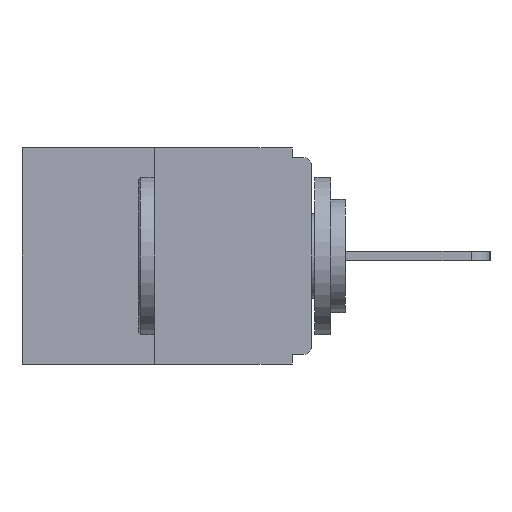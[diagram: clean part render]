
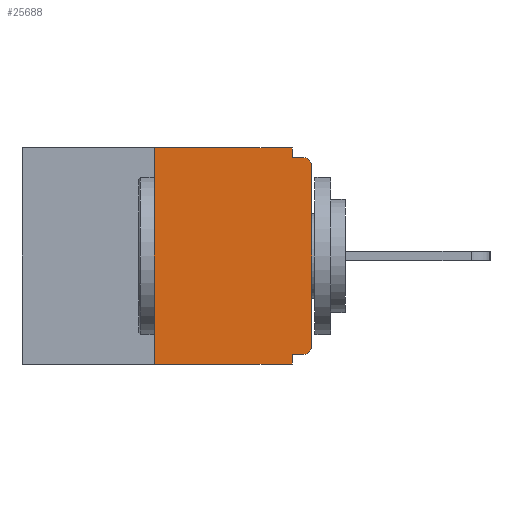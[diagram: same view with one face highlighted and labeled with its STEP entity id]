
A CAD part, left-side view. The second image highlights one B-rep face of the part: STEP entity #25688.
In plain terms, the highlighted planar face has unit normal (-1, 0, 0).
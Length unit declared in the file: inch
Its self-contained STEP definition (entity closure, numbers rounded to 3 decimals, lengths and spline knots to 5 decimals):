
#72 = DIRECTION ( 'NONE',  ( 0., 0., -1. ) ) ;
#695 = CARTESIAN_POINT ( 'NONE',  ( 0., 0.25, -0.343 ) ) ;
#706 = ORIENTED_EDGE ( 'NONE', *, *, #8228, .T. ) ;
#1074 = ORIENTED_EDGE ( 'NONE', *, *, #24626, .F. ) ;
#1727 = LINE ( 'NONE', #18703, #23089 ) ;
#2101 = DIRECTION ( 'NONE',  ( -1., 0., 0. ) ) ;
#2725 = DIRECTION ( 'NONE',  ( 0., -1., 0. ) ) ;
#3169 = DIRECTION ( 'NONE',  ( 0., -1., 0. ) ) ;
#3183 = AXIS2_PLACEMENT_3D ( 'NONE', #14645, #2101, #16706 ) ;
#3977 = DIRECTION ( 'NONE',  ( 0., 0., -1. ) ) ;
#4123 = VERTEX_POINT ( 'NONE', #26659 ) ;
#4604 = VERTEX_POINT ( 'NONE', #12028 ) ;
#4611 = CARTESIAN_POINT ( 'NONE',  ( 0., 0.46, 0. ) ) ;
#4741 = VERTEX_POINT ( 'NONE', #11753 ) ;
#4864 = CARTESIAN_POINT ( 'NONE',  ( 0., 0., -0.015 ) ) ;
#5472 = CIRCLE ( 'NONE', #3183, 0.015 ) ;
#5597 = CARTESIAN_POINT ( 'NONE',  ( 0., 0.031, 0. ) ) ;
#5767 = VERTEX_POINT ( 'NONE', #5597 ) ;
#6042 = VECTOR ( 'NONE', #9675, 39.37008 ) ;
#6302 = EDGE_CURVE ( 'NONE', #8585, #10122, #25726, .T. ) ;
#6752 = DIRECTION ( 'NONE',  ( 0., 0., -1. ) ) ;
#6762 = VERTEX_POINT ( 'NONE', #8895 ) ;
#6988 = VERTEX_POINT ( 'NONE', #695 ) ;
#7781 = ORIENTED_EDGE ( 'NONE', *, *, #11157, .F. ) ;
#7990 = LINE ( 'NONE', #4864, #12855 ) ;
#8228 = EDGE_CURVE ( 'NONE', #6762, #8585, #5472, .T. ) ;
#8324 = CIRCLE ( 'NONE', #12993, 0.015 ) ;
#8351 = VECTOR ( 'NONE', #23105, 39.37008 ) ;
#8444 = DIRECTION ( 'NONE',  ( 0., 0., 1. ) ) ;
#8585 = VERTEX_POINT ( 'NONE', #9466 ) ;
#8895 = CARTESIAN_POINT ( 'NONE',  ( 0., 0.015, -0.328 ) ) ;
#9466 = CARTESIAN_POINT ( 'NONE',  ( 0., 0., -0.313 ) ) ;
#9675 = DIRECTION ( 'NONE',  ( 0., -1., 0. ) ) ;
#9811 = ORIENTED_EDGE ( 'NONE', *, *, #11003, .F. ) ;
#9943 = EDGE_CURVE ( 'NONE', #4741, #5767, #11579, .T. ) ;
#10122 = VERTEX_POINT ( 'NONE', #24546 ) ;
#10159 = VECTOR ( 'NONE', #23240, 39.37008 ) ;
#10326 = VECTOR ( 'NONE', #3977, 39.37008 ) ;
#10464 = ORIENTED_EDGE ( 'NONE', *, *, #9943, .F. ) ;
#11003 = EDGE_CURVE ( 'NONE', #4123, #4604, #7990, .T. ) ;
#11023 = ORIENTED_EDGE ( 'NONE', *, *, #12562, .F. ) ;
#11157 = EDGE_CURVE ( 'NONE', #5767, #4123, #12655, .T. ) ;
#11325 = ORIENTED_EDGE ( 'NONE', *, *, #6302, .T. ) ;
#11579 = LINE ( 'NONE', #15812, #6042 ) ;
#11619 = DIRECTION ( 'NONE',  ( 0., 0., -1. ) ) ;
#11623 = VERTEX_POINT ( 'NONE', #13139 ) ;
#11753 = CARTESIAN_POINT ( 'NONE',  ( 0., 0.25, 0. ) ) ;
#12028 = CARTESIAN_POINT ( 'NONE',  ( 0., 0.015, -0.015 ) ) ;
#12517 = ORIENTED_EDGE ( 'NONE', *, *, #25113, .T. ) ;
#12562 = EDGE_CURVE ( 'NONE', #11623, #21097, #21259, .T. ) ;
#12655 = LINE ( 'NONE', #25777, #18104 ) ;
#12779 = DIRECTION ( 'NONE',  ( -1., 0., 0. ) ) ;
#12827 = FACE_OUTER_BOUND ( 'NONE', #16823, .T. ) ;
#12855 = VECTOR ( 'NONE', #2725, 39.37008 ) ;
#12993 = AXIS2_PLACEMENT_3D ( 'NONE', #24896, #12779, #72 ) ;
#13139 = CARTESIAN_POINT ( 'NONE',  ( 0., 0.031, -0.328 ) ) ;
#14645 = CARTESIAN_POINT ( 'NONE',  ( 0., 0.015, -0.313 ) ) ;
#15122 = LINE ( 'NONE', #23185, #8351 ) ;
#15241 = ORIENTED_EDGE ( 'NONE', *, *, #19416, .F. ) ;
#15812 = CARTESIAN_POINT ( 'NONE',  ( 0., 0.46, 0. ) ) ;
#15843 = CARTESIAN_POINT ( 'NONE',  ( 0., 0.031, -0.343 ) ) ;
#15960 = CARTESIAN_POINT ( 'NONE',  ( 0., 0.031, -0.343 ) ) ;
#16706 = DIRECTION ( 'NONE',  ( 0., 0., -1. ) ) ;
#16823 = EDGE_LOOP ( 'NONE', ( #10464, #15241, #17337, #11023, #1074, #706, #11325, #12517, #9811, #7781 ) ) ;
#16956 = PLANE ( 'NONE',  #17453 ) ;
#17337 = ORIENTED_EDGE ( 'NONE', *, *, #18049, .T. ) ;
#17453 = AXIS2_PLACEMENT_3D ( 'NONE', #4611, #19089, #6752 ) ;
#17704 = CARTESIAN_POINT ( 'NONE',  ( 0., 0.46, -0.343 ) ) ;
#18049 = EDGE_CURVE ( 'NONE', #6988, #21097, #25017, .T. ) ;
#18104 = VECTOR ( 'NONE', #11619, 39.37008 ) ;
#18703 = CARTESIAN_POINT ( 'NONE',  ( 0., 0.25, 0. ) ) ;
#19089 = DIRECTION ( 'NONE',  ( 1., 0., 0. ) ) ;
#19416 = EDGE_CURVE ( 'NONE', #6988, #4741, #1727, .T. ) ;
#21097 = VERTEX_POINT ( 'NONE', #15843 ) ;
#21259 = LINE ( 'NONE', #15960, #10326 ) ;
#23089 = VECTOR ( 'NONE', #8444, 39.37008 ) ;
#23105 = DIRECTION ( 'NONE',  ( 0., 1., 0. ) ) ;
#23185 = CARTESIAN_POINT ( 'NONE',  ( 0., 0., -0.328 ) ) ;
#23240 = DIRECTION ( 'NONE',  ( 0., 0., 1. ) ) ;
#23580 = CARTESIAN_POINT ( 'NONE',  ( 0., 0., 0. ) ) ;
#24546 = CARTESIAN_POINT ( 'NONE',  ( 0., 0., -0.03 ) ) ;
#24626 = EDGE_CURVE ( 'NONE', #6762, #11623, #15122, .T. ) ;
#24896 = CARTESIAN_POINT ( 'NONE',  ( 0., 0.015, -0.03 ) ) ;
#25017 = LINE ( 'NONE', #17704, #25642 ) ;
#25113 = EDGE_CURVE ( 'NONE', #10122, #4604, #8324, .T. ) ;
#25642 = VECTOR ( 'NONE', #3169, 39.37008 ) ;
#25688 = ADVANCED_FACE ( 'NONE', ( #12827 ), #16956, .F. ) ;
#25726 = LINE ( 'NONE', #23580, #10159 ) ;
#25777 = CARTESIAN_POINT ( 'NONE',  ( 0., 0.031, 0. ) ) ;
#26659 = CARTESIAN_POINT ( 'NONE',  ( 0., 0.031, -0.015 ) ) ;
